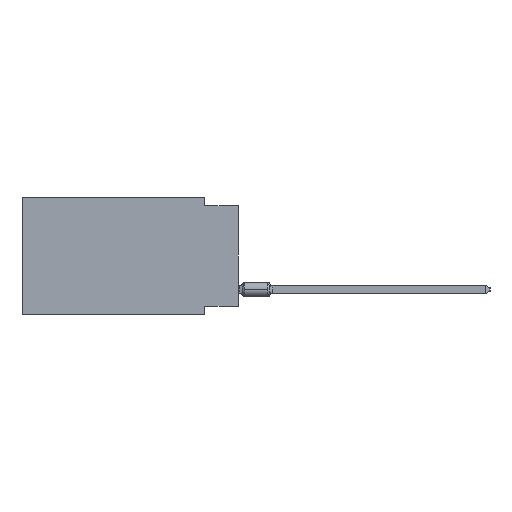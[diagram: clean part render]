
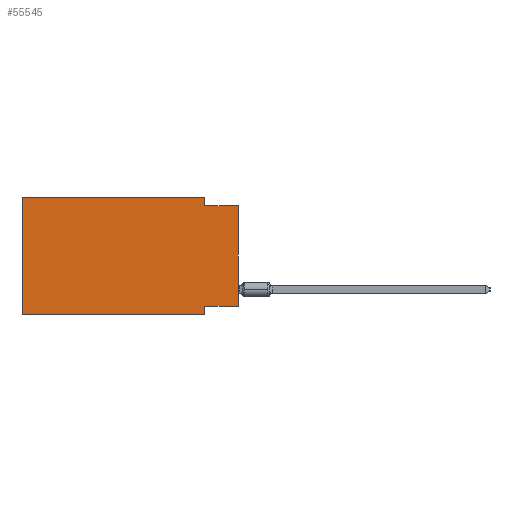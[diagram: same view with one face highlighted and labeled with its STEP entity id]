
A CAD part, left-side view. The second image highlights one B-rep face of the part: STEP entity #55545.
In plain terms, the highlighted planar face has unit normal (-1, 0, 0).
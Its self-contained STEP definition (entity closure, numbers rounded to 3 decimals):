
#2024 = ORIENTED_EDGE ( 'NONE', *, *, #4898, .F. ) ;
#3777 = CARTESIAN_POINT ( 'NONE',  ( 0., 0., 0. ) ) ;
#4898 = EDGE_CURVE ( 'NONE', #20888, #53858, #56909, .T. ) ;
#5668 = EDGE_CURVE ( 'NONE', #30701, #73283, #29765, .T. ) ;
#6236 = LINE ( 'NONE', #41252, #76585 ) ;
#6753 = CARTESIAN_POINT ( 'NONE',  ( 0., 0., -0.635 ) ) ;
#6984 = EDGE_CURVE ( 'NONE', #18429, #43315, #37636, .T. ) ;
#7230 = ORIENTED_EDGE ( 'NONE', *, *, #24001, .F. ) ;
#9895 = CARTESIAN_POINT ( 'NONE',  ( 0., 2.54, 0. ) ) ;
#10878 = EDGE_LOOP ( 'NONE', ( #69445, #22134, #2024, #57759, #16155, #74063, #7230, #44179 ) ) ;
#11121 = DIRECTION ( 'NONE',  ( 0., 0., -1. ) ) ;
#11144 = VECTOR ( 'NONE', #56686, 1000. ) ;
#12535 = DIRECTION ( 'NONE',  ( 0., -1., 0. ) ) ;
#13016 = VECTOR ( 'NONE', #27701, 1000. ) ;
#13312 = LINE ( 'NONE', #55365, #52280 ) ;
#13587 = CARTESIAN_POINT ( 'NONE',  ( 0., 16.383, -8.89 ) ) ;
#15053 = DIRECTION ( 'NONE',  ( 0., 0., 1. ) ) ;
#16155 = ORIENTED_EDGE ( 'NONE', *, *, #5668, .F. ) ;
#16367 = DIRECTION ( 'NONE',  ( 0., -1., 0. ) ) ;
#18176 = EDGE_CURVE ( 'NONE', #30701, #73831, #13312, .T. ) ;
#18429 = VERTEX_POINT ( 'NONE', #65004 ) ;
#19321 = AXIS2_PLACEMENT_3D ( 'NONE', #38277, #38657, #62792 ) ;
#20115 = LINE ( 'NONE', #61763, #11144 ) ;
#20839 = VECTOR ( 'NONE', #44801, 1000. ) ;
#20888 = VERTEX_POINT ( 'NONE', #9895 ) ;
#21737 = EDGE_CURVE ( 'NONE', #73283, #20888, #33887, .T. ) ;
#22134 = ORIENTED_EDGE ( 'NONE', *, *, #40348, .F. ) ;
#23171 = CARTESIAN_POINT ( 'NONE',  ( 0., 16.383, 0. ) ) ;
#24001 = EDGE_CURVE ( 'NONE', #45298, #73831, #46926, .T. ) ;
#26528 = CARTESIAN_POINT ( 'NONE',  ( 0., 2.54, -8.255 ) ) ;
#27701 = DIRECTION ( 'NONE',  ( 0., 0., -1. ) ) ;
#29765 = LINE ( 'NONE', #23171, #75203 ) ;
#30701 = VERTEX_POINT ( 'NONE', #13587 ) ;
#32367 = EDGE_CURVE ( 'NONE', #18429, #45298, #20115, .T. ) ;
#33887 = LINE ( 'NONE', #57636, #20839 ) ;
#33961 = CARTESIAN_POINT ( 'NONE',  ( 0., 16.383, 0. ) ) ;
#34615 = CARTESIAN_POINT ( 'NONE',  ( 0., 2.54, -8.89 ) ) ;
#37636 = LINE ( 'NONE', #3777, #74153 ) ;
#38277 = CARTESIAN_POINT ( 'NONE',  ( 0., 16.383, 0. ) ) ;
#38657 = DIRECTION ( 'NONE',  ( 1., 0., 0. ) ) ;
#38990 = CARTESIAN_POINT ( 'NONE',  ( 0., 2.54, 0. ) ) ;
#39505 = CARTESIAN_POINT ( 'NONE',  ( 0., 2.54, -0.635 ) ) ;
#40348 = EDGE_CURVE ( 'NONE', #53858, #43315, #6236, .T. ) ;
#41247 = VECTOR ( 'NONE', #11121, 1000. ) ;
#41252 = CARTESIAN_POINT ( 'NONE',  ( 0., 0., -0.635 ) ) ;
#43315 = VERTEX_POINT ( 'NONE', #6753 ) ;
#44179 = ORIENTED_EDGE ( 'NONE', *, *, #32367, .F. ) ;
#44801 = DIRECTION ( 'NONE',  ( 0., -1., 0. ) ) ;
#45298 = VERTEX_POINT ( 'NONE', #26528 ) ;
#46926 = LINE ( 'NONE', #64815, #41247 ) ;
#52280 = VECTOR ( 'NONE', #12535, 1000. ) ;
#53858 = VERTEX_POINT ( 'NONE', #39505 ) ;
#55365 = CARTESIAN_POINT ( 'NONE',  ( 0., 16.383, -8.89 ) ) ;
#55545 = ADVANCED_FACE ( 'NONE', ( #68241 ), #73703, .F. ) ;
#56686 = DIRECTION ( 'NONE',  ( 0., 1., 0. ) ) ;
#56909 = LINE ( 'NONE', #38990, #13016 ) ;
#57636 = CARTESIAN_POINT ( 'NONE',  ( 0., 16.383, 0. ) ) ;
#57759 = ORIENTED_EDGE ( 'NONE', *, *, #21737, .F. ) ;
#60113 = DIRECTION ( 'NONE',  ( 0., 0., 1. ) ) ;
#61763 = CARTESIAN_POINT ( 'NONE',  ( 0., 0., -8.255 ) ) ;
#62792 = DIRECTION ( 'NONE',  ( 0., 0., -1. ) ) ;
#64815 = CARTESIAN_POINT ( 'NONE',  ( 0., 2.54, -8.89 ) ) ;
#65004 = CARTESIAN_POINT ( 'NONE',  ( 0., 0., -8.255 ) ) ;
#68241 = FACE_OUTER_BOUND ( 'NONE', #10878, .T. ) ;
#69445 = ORIENTED_EDGE ( 'NONE', *, *, #6984, .T. ) ;
#73283 = VERTEX_POINT ( 'NONE', #33961 ) ;
#73703 = PLANE ( 'NONE',  #19321 ) ;
#73831 = VERTEX_POINT ( 'NONE', #34615 ) ;
#74063 = ORIENTED_EDGE ( 'NONE', *, *, #18176, .T. ) ;
#74153 = VECTOR ( 'NONE', #15053, 1000. ) ;
#75203 = VECTOR ( 'NONE', #60113, 1000. ) ;
#76585 = VECTOR ( 'NONE', #16367, 1000. ) ;
